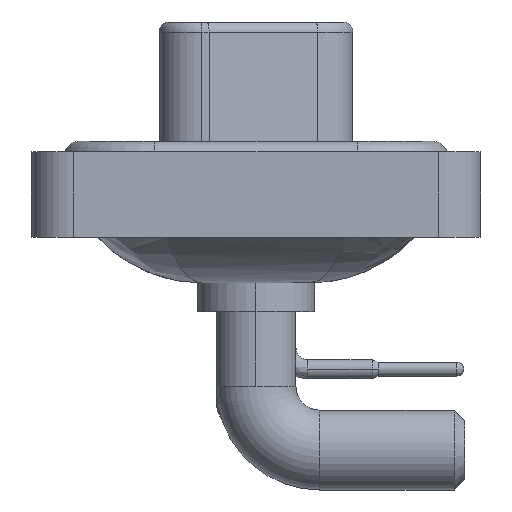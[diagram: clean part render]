
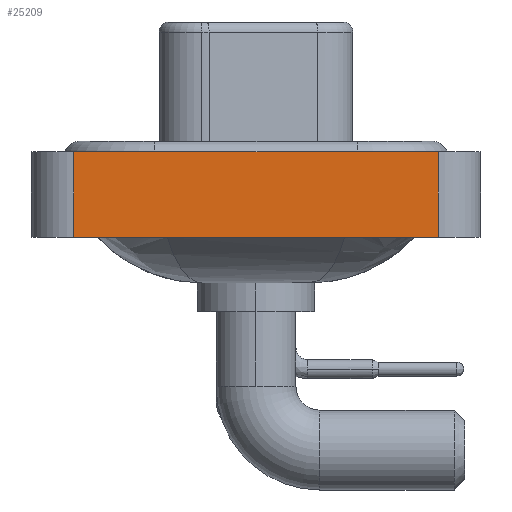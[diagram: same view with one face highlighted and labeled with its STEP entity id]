
A CAD part, left-side view. The second image highlights one B-rep face of the part: STEP entity #25209.
In plain terms, the highlighted planar face has unit normal (-1, 0, 0).
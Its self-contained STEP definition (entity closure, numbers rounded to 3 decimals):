
#599 = VERTEX_POINT ( 'NONE', #6524 ) ;
#715 = DIRECTION ( 'NONE',  ( 0., -1., 0. ) ) ;
#1214 = CARTESIAN_POINT ( 'NONE',  ( -7.35, 8.55, -3.6 ) ) ;
#1687 = CARTESIAN_POINT ( 'NONE',  ( -7.35, -8.55, 0.4 ) ) ;
#3814 = EDGE_CURVE ( 'NONE', #599, #15321, #23815, .T. ) ;
#3882 = CARTESIAN_POINT ( 'NONE',  ( -7.35, 8.55, 0.4 ) ) ;
#5423 = LINE ( 'NONE', #1214, #20794 ) ;
#5447 = DIRECTION ( 'NONE',  ( 0., 0., 1. ) ) ;
#5939 = VERTEX_POINT ( 'NONE', #17782 ) ;
#6524 = CARTESIAN_POINT ( 'NONE',  ( -7.35, -8.55, -3.6 ) ) ;
#8418 = CARTESIAN_POINT ( 'NONE',  ( -7.35, -8.55, 0.4 ) ) ;
#9649 = DIRECTION ( 'NONE',  ( 0., 0., 1. ) ) ;
#9788 = DIRECTION ( 'NONE',  ( -1., 0., 0. ) ) ;
#9839 = EDGE_LOOP ( 'NONE', ( #16505, #24977, #23918, #13522 ) ) ;
#10518 = VECTOR ( 'NONE', #5447, 1000. ) ;
#11371 = FACE_OUTER_BOUND ( 'NONE', #9839, .T. ) ;
#13522 = ORIENTED_EDGE ( 'NONE', *, *, #24696, .T. ) ;
#13853 = CARTESIAN_POINT ( 'NONE',  ( -7.35, -8.55, -3.6 ) ) ;
#14324 = DIRECTION ( 'NONE',  ( 0., -1., 0. ) ) ;
#15321 = VERTEX_POINT ( 'NONE', #8418 ) ;
#16505 = ORIENTED_EDGE ( 'NONE', *, *, #3814, .T. ) ;
#17437 = VECTOR ( 'NONE', #715, 1000. ) ;
#17782 = CARTESIAN_POINT ( 'NONE',  ( -7.35, 8.55, -3.6 ) ) ;
#19537 = DIRECTION ( 'NONE',  ( 0., 0., 1. ) ) ;
#19749 = LINE ( 'NONE', #1687, #21930 ) ;
#19936 = EDGE_CURVE ( 'NONE', #21701, #15321, #19749, .T. ) ;
#20771 = CARTESIAN_POINT ( 'NONE',  ( -7.35, -8.55, -3.6 ) ) ;
#20794 = VECTOR ( 'NONE', #19537, 1000. ) ;
#21237 = AXIS2_PLACEMENT_3D ( 'NONE', #13853, #9788, #9649 ) ;
#21701 = VERTEX_POINT ( 'NONE', #3882 ) ;
#21930 = VECTOR ( 'NONE', #14324, 1000. ) ;
#23815 = LINE ( 'NONE', #25263, #10518 ) ;
#23918 = ORIENTED_EDGE ( 'NONE', *, *, #24226, .F. ) ;
#24226 = EDGE_CURVE ( 'NONE', #5939, #21701, #5423, .T. ) ;
#24696 = EDGE_CURVE ( 'NONE', #5939, #599, #25272, .T. ) ;
#24977 = ORIENTED_EDGE ( 'NONE', *, *, #19936, .F. ) ;
#25209 = ADVANCED_FACE ( 'NONE', ( #11371 ), #25887, .T. ) ;
#25263 = CARTESIAN_POINT ( 'NONE',  ( -7.35, -8.55, -3.6 ) ) ;
#25272 = LINE ( 'NONE', #20771, #17437 ) ;
#25887 = PLANE ( 'NONE',  #21237 ) ;
